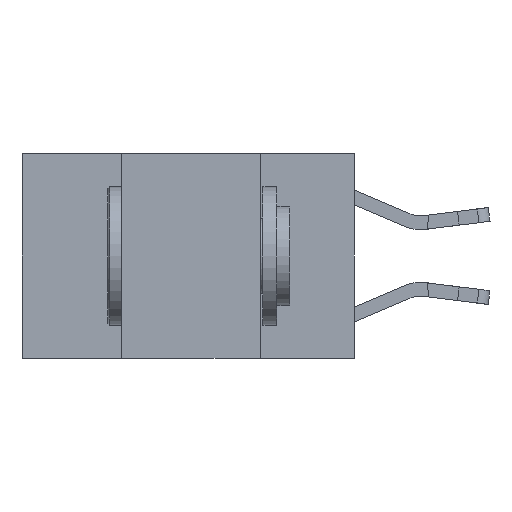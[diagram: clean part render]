
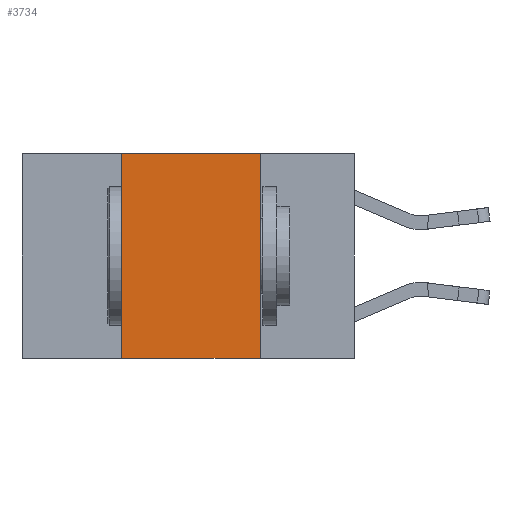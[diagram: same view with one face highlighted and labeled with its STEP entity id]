
A CAD part, left-side view. The second image highlights one B-rep face of the part: STEP entity #3734.
In plain terms, the highlighted planar face has unit normal (-1, 0, 0).
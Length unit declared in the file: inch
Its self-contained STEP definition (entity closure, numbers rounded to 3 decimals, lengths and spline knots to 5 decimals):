
#34 = CARTESIAN_POINT ( 'NONE',  ( 0., 0.6, -0.37 ) ) ;
#93 = DIRECTION ( 'NONE',  ( 0., -1., 0. ) ) ;
#441 = CARTESIAN_POINT ( 'NONE',  ( 0., 0.17, -0.37 ) ) ;
#588 = LINE ( 'NONE', #7614, #8059 ) ;
#787 = VERTEX_POINT ( 'NONE', #7691 ) ;
#1161 = VECTOR ( 'NONE', #9726, 39.37008 ) ;
#1561 = CARTESIAN_POINT ( 'NONE',  ( 0., 0.42, 0. ) ) ;
#2195 = EDGE_CURVE ( 'NONE', #12384, #787, #14422, .T. ) ;
#2539 = ORIENTED_EDGE ( 'NONE', *, *, #2195, .F. ) ;
#2642 = VECTOR ( 'NONE', #93, 39.37008 ) ;
#2837 = LINE ( 'NONE', #9496, #1161 ) ;
#3487 = VECTOR ( 'NONE', #14369, 39.37008 ) ;
#3734 = ADVANCED_FACE ( 'NONE', ( #6264 ), #4114, .F. ) ;
#3970 = ORIENTED_EDGE ( 'NONE', *, *, #13113, .F. ) ;
#4046 = CARTESIAN_POINT ( 'NONE',  ( 0., 0.6, 0. ) ) ;
#4114 = PLANE ( 'NONE',  #8836 ) ;
#5141 = DIRECTION ( 'NONE',  ( 1., 0., 0. ) ) ;
#5842 = EDGE_CURVE ( 'NONE', #6529, #9840, #7721, .T. ) ;
#6112 = ORIENTED_EDGE ( 'NONE', *, *, #5842, .T. ) ;
#6264 = FACE_OUTER_BOUND ( 'NONE', #9092, .T. ) ;
#6529 = VERTEX_POINT ( 'NONE', #8426 ) ;
#7384 = DIRECTION ( 'NONE',  ( 0., 0., 1. ) ) ;
#7455 = ORIENTED_EDGE ( 'NONE', *, *, #8794, .F. ) ;
#7614 = CARTESIAN_POINT ( 'NONE',  ( 0., 0.42, 0. ) ) ;
#7691 = CARTESIAN_POINT ( 'NONE',  ( 0., 0.17, 0. ) ) ;
#7721 = LINE ( 'NONE', #34, #3487 ) ;
#8059 = VECTOR ( 'NONE', #7384, 39.37008 ) ;
#8426 = CARTESIAN_POINT ( 'NONE',  ( 0., 0.42, -0.37 ) ) ;
#8604 = DIRECTION ( 'NONE',  ( 0., 0., -1. ) ) ;
#8794 = EDGE_CURVE ( 'NONE', #787, #9840, #2837, .T. ) ;
#8836 = AXIS2_PLACEMENT_3D ( 'NONE', #4046, #5141, #8604 ) ;
#9092 = EDGE_LOOP ( 'NONE', ( #7455, #2539, #3970, #6112 ) ) ;
#9496 = CARTESIAN_POINT ( 'NONE',  ( 0., 0.17, 0. ) ) ;
#9726 = DIRECTION ( 'NONE',  ( 0., 0., -1. ) ) ;
#9840 = VERTEX_POINT ( 'NONE', #441 ) ;
#11173 = CARTESIAN_POINT ( 'NONE',  ( 0., 0.6, 0. ) ) ;
#12384 = VERTEX_POINT ( 'NONE', #1561 ) ;
#13113 = EDGE_CURVE ( 'NONE', #6529, #12384, #588, .T. ) ;
#14369 = DIRECTION ( 'NONE',  ( 0., -1., 0. ) ) ;
#14422 = LINE ( 'NONE', #11173, #2642 ) ;
